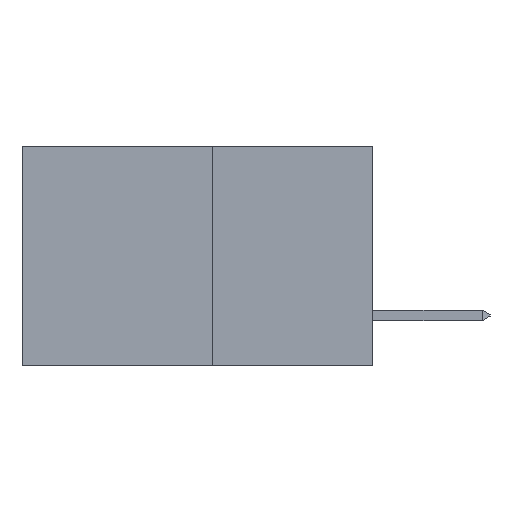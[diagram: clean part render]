
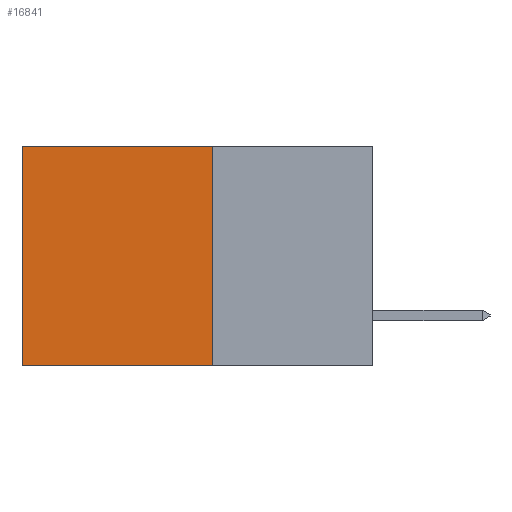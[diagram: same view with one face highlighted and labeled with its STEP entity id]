
A CAD part, left-side view. The second image highlights one B-rep face of the part: STEP entity #16841.
In plain terms, the highlighted planar face has unit normal (-1, 0, 0).
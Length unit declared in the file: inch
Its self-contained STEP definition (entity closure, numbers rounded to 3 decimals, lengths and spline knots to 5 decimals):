
#112 = VECTOR ( 'NONE', #396, 39.37008 ) ;
#382 = EDGE_CURVE ( 'NONE', #6166, #3569, #15836, .T. ) ;
#396 = DIRECTION ( 'NONE',  ( 0., 0., -1. ) ) ;
#1872 = ORIENTED_EDGE ( 'NONE', *, *, #382, .F. ) ;
#2388 = DIRECTION ( 'NONE',  ( 0., 0., -1. ) ) ;
#2622 = VECTOR ( 'NONE', #3348, 39.37008 ) ;
#3005 = EDGE_CURVE ( 'NONE', #10442, #3569, #8005, .T. ) ;
#3348 = DIRECTION ( 'NONE',  ( 0., 1., 0. ) ) ;
#3371 = CARTESIAN_POINT ( 'NONE',  ( 0.277, 0.27, 0. ) ) ;
#3569 = VERTEX_POINT ( 'NONE', #16856 ) ;
#4130 = EDGE_CURVE ( 'NONE', #6887, #6166, #8565, .T. ) ;
#5680 = PLANE ( 'NONE',  #10470 ) ;
#6166 = VERTEX_POINT ( 'NONE', #13985 ) ;
#6407 = ORIENTED_EDGE ( 'NONE', *, *, #4130, .F. ) ;
#6887 = VERTEX_POINT ( 'NONE', #16285 ) ;
#7113 = DIRECTION ( 'NONE',  ( 0., 0., -1. ) ) ;
#7157 = CARTESIAN_POINT ( 'NONE',  ( 0.277, 0.27, -0.37 ) ) ;
#8005 = LINE ( 'NONE', #8535, #14947 ) ;
#8047 = EDGE_CURVE ( 'NONE', #6887, #10442, #16748, .T. ) ;
#8535 = CARTESIAN_POINT ( 'NONE',  ( 0.277, 0.59, -0.37 ) ) ;
#8565 = LINE ( 'NONE', #7157, #112 ) ;
#9008 = FACE_OUTER_BOUND ( 'NONE', #16400, .T. ) ;
#9343 = ORIENTED_EDGE ( 'NONE', *, *, #8047, .T. ) ;
#10238 = DIRECTION ( 'NONE',  ( 0., 1., 0. ) ) ;
#10442 = VERTEX_POINT ( 'NONE', #15020 ) ;
#10470 = AXIS2_PLACEMENT_3D ( 'NONE', #11039, #14895, #7113 ) ;
#11039 = CARTESIAN_POINT ( 'NONE',  ( 0.277, 0.27, -0.37 ) ) ;
#12465 = VECTOR ( 'NONE', #10238, 39.37008 ) ;
#12700 = CARTESIAN_POINT ( 'NONE',  ( 0.277, 0.27, -0.37 ) ) ;
#13985 = CARTESIAN_POINT ( 'NONE',  ( 0.277, 0.27, -0.37 ) ) ;
#14895 = DIRECTION ( 'NONE',  ( 1., 0., 0. ) ) ;
#14947 = VECTOR ( 'NONE', #2388, 39.37008 ) ;
#15020 = CARTESIAN_POINT ( 'NONE',  ( 0.277, 0.59, 0. ) ) ;
#15836 = LINE ( 'NONE', #12700, #12465 ) ;
#16285 = CARTESIAN_POINT ( 'NONE',  ( 0.277, 0.27, 0. ) ) ;
#16400 = EDGE_LOOP ( 'NONE', ( #17489, #1872, #6407, #9343 ) ) ;
#16748 = LINE ( 'NONE', #3371, #2622 ) ;
#16841 = ADVANCED_FACE ( 'NONE', ( #9008 ), #5680, .F. ) ;
#16856 = CARTESIAN_POINT ( 'NONE',  ( 0.277, 0.59, -0.37 ) ) ;
#17489 = ORIENTED_EDGE ( 'NONE', *, *, #3005, .T. ) ;
